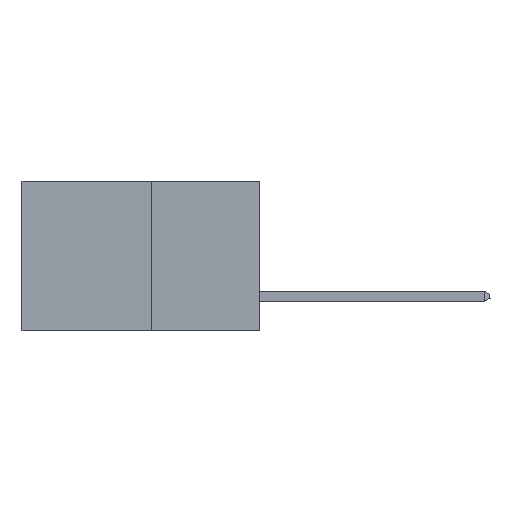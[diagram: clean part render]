
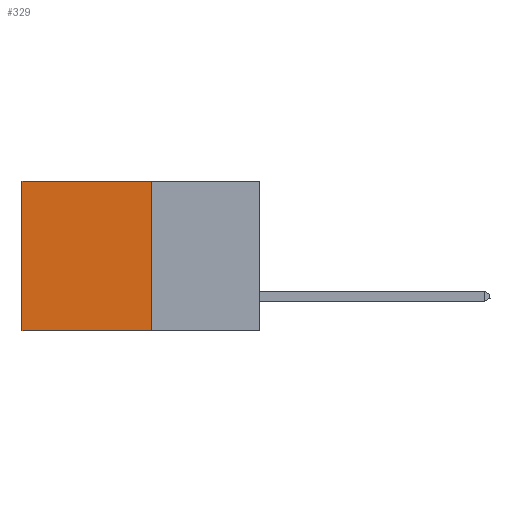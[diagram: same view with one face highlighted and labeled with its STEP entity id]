
A CAD part, left-side view. The second image highlights one B-rep face of the part: STEP entity #329.
In plain terms, the highlighted planar face has unit normal (-1, 0, 0).
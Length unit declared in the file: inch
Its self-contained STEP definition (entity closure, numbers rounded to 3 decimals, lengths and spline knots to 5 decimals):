
#116 = LINE ( 'NONE', #17227, #26566 ) ;
#160 = CARTESIAN_POINT ( 'NONE',  ( 0.277, 0.27, -0.37 ) ) ;
#189 = DIRECTION ( 'NONE',  ( 0., 1., 0. ) ) ;
#219 = DIRECTION ( 'NONE',  ( 0., 0., -1. ) ) ;
#261 = DIRECTION ( 'NONE',  ( 1., 0., 0. ) ) ;
#329 = ADVANCED_FACE ( 'NONE', ( #10017 ), #6423, .F. ) ;
#2682 = VECTOR ( 'NONE', #2807, 39.37008 ) ;
#2807 = DIRECTION ( 'NONE',  ( 0., 0., -1. ) ) ;
#3527 = VERTEX_POINT ( 'NONE', #6495 ) ;
#4255 = AXIS2_PLACEMENT_3D ( 'NONE', #160, #261, #219 ) ;
#5281 = VERTEX_POINT ( 'NONE', #9485 ) ;
#5452 = LINE ( 'NONE', #8997, #26865 ) ;
#6157 = CARTESIAN_POINT ( 'NONE',  ( 0.277, 0.27, -0.37 ) ) ;
#6239 = VERTEX_POINT ( 'NONE', #6157 ) ;
#6423 = PLANE ( 'NONE',  #4255 ) ;
#6495 = CARTESIAN_POINT ( 'NONE',  ( 0.277, 0.27, 0. ) ) ;
#6761 = DIRECTION ( 'NONE',  ( 0., 1., 0. ) ) ;
#7973 = ORIENTED_EDGE ( 'NONE', *, *, #8754, .T. ) ;
#8195 = EDGE_LOOP ( 'NONE', ( #9946, #19378, #13394, #7973 ) ) ;
#8754 = EDGE_CURVE ( 'NONE', #3527, #5281, #116, .T. ) ;
#8997 = CARTESIAN_POINT ( 'NONE',  ( 0.277, 0.27, -0.37 ) ) ;
#9485 = CARTESIAN_POINT ( 'NONE',  ( 0.277, 0.59, 0. ) ) ;
#9946 = ORIENTED_EDGE ( 'NONE', *, *, #10788, .T. ) ;
#10017 = FACE_OUTER_BOUND ( 'NONE', #8195, .T. ) ;
#10788 = EDGE_CURVE ( 'NONE', #5281, #16269, #14087, .T. ) ;
#13107 = CARTESIAN_POINT ( 'NONE',  ( 0.277, 0.27, -0.37 ) ) ;
#13117 = VECTOR ( 'NONE', #6761, 39.37008 ) ;
#13394 = ORIENTED_EDGE ( 'NONE', *, *, #18852, .F. ) ;
#14087 = LINE ( 'NONE', #15624, #2682 ) ;
#15624 = CARTESIAN_POINT ( 'NONE',  ( 0.277, 0.59, -0.37 ) ) ;
#16269 = VERTEX_POINT ( 'NONE', #26294 ) ;
#17227 = CARTESIAN_POINT ( 'NONE',  ( 0.277, 0.27, 0. ) ) ;
#17411 = DIRECTION ( 'NONE',  ( 0., 0., -1. ) ) ;
#18815 = LINE ( 'NONE', #13107, #13117 ) ;
#18852 = EDGE_CURVE ( 'NONE', #3527, #6239, #5452, .T. ) ;
#19378 = ORIENTED_EDGE ( 'NONE', *, *, #20539, .F. ) ;
#20539 = EDGE_CURVE ( 'NONE', #6239, #16269, #18815, .T. ) ;
#26294 = CARTESIAN_POINT ( 'NONE',  ( 0.277, 0.59, -0.37 ) ) ;
#26566 = VECTOR ( 'NONE', #189, 39.37008 ) ;
#26865 = VECTOR ( 'NONE', #17411, 39.37008 ) ;
